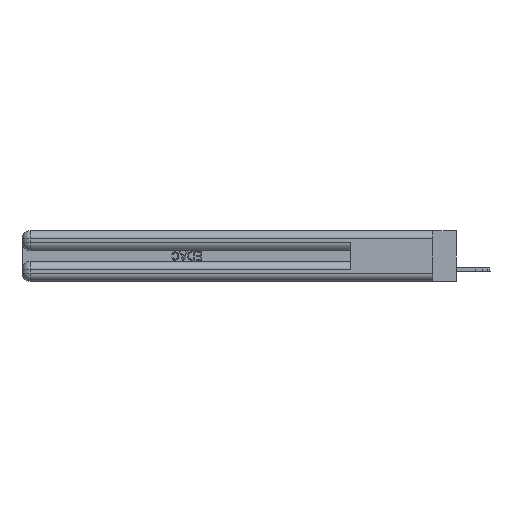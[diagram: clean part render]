
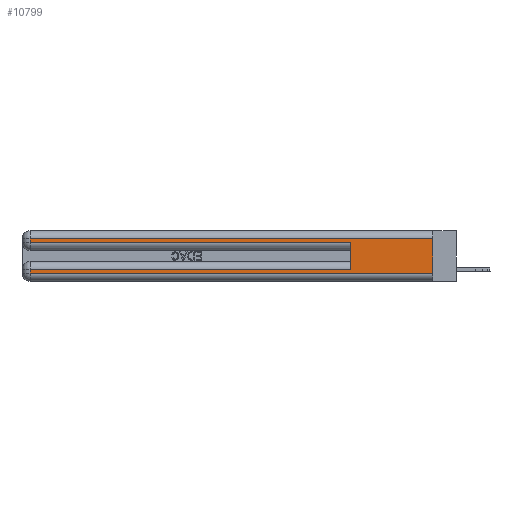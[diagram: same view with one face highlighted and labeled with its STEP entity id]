
A CAD part, left-side view. The second image highlights one B-rep face of the part: STEP entity #10799.
In plain terms, the highlighted planar face has unit normal (-1, 0, 0).
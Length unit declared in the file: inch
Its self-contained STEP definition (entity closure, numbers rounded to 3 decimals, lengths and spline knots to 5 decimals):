
#1402 = LINE ( 'NONE', #39074, #12026 ) ;
#1666 = ORIENTED_EDGE ( 'NONE', *, *, #37206, .F. ) ;
#1807 = PLANE ( 'NONE',  #17570 ) ;
#2458 = CARTESIAN_POINT ( 'NONE',  ( 0., 2.94, 0.06 ) ) ;
#2576 = CARTESIAN_POINT ( 'NONE',  ( 0., 0., 0.31 ) ) ;
#3632 = CARTESIAN_POINT ( 'NONE',  ( 0., 0., 0.085 ) ) ;
#4498 = LINE ( 'NONE', #38689, #5993 ) ;
#5146 = ORIENTED_EDGE ( 'NONE', *, *, #19513, .F. ) ;
#5199 = VERTEX_POINT ( 'NONE', #5343 ) ;
#5343 = CARTESIAN_POINT ( 'NONE',  ( 0., 2.94, 0.085 ) ) ;
#5422 = CARTESIAN_POINT ( 'NONE',  ( 0., 0., 0.37 ) ) ;
#5439 = ORIENTED_EDGE ( 'NONE', *, *, #12116, .T. ) ;
#5514 = CARTESIAN_POINT ( 'NONE',  ( 0., 0., 0.285 ) ) ;
#5993 = VECTOR ( 'NONE', #23153, 39.37008 ) ;
#6427 = VECTOR ( 'NONE', #16895, 39.37008 ) ;
#7506 = CARTESIAN_POINT ( 'NONE',  ( 0., 0., 0.31 ) ) ;
#7989 = DIRECTION ( 'NONE',  ( 0., 1., 0. ) ) ;
#9188 = VERTEX_POINT ( 'NONE', #35377 ) ;
#9248 = LINE ( 'NONE', #5422, #35304 ) ;
#9866 = VERTEX_POINT ( 'NONE', #32446 ) ;
#10028 = VECTOR ( 'NONE', #38394, 39.37008 ) ;
#10799 = ADVANCED_FACE ( 'NONE', ( #15548 ), #1807, .F. ) ;
#11138 = LINE ( 'NONE', #32343, #25615 ) ;
#12018 = VERTEX_POINT ( 'NONE', #26527 ) ;
#12026 = VECTOR ( 'NONE', #39212, 39.37008 ) ;
#12116 = EDGE_CURVE ( 'NONE', #9188, #5199, #19333, .T. ) ;
#13262 = VERTEX_POINT ( 'NONE', #38378 ) ;
#13413 = EDGE_CURVE ( 'NONE', #35289, #13262, #34206, .T. ) ;
#14549 = VERTEX_POINT ( 'NONE', #2458 ) ;
#14654 = DIRECTION ( 'NONE',  ( 0., 0., -1. ) ) ;
#15548 = FACE_OUTER_BOUND ( 'NONE', #35232, .T. ) ;
#16895 = DIRECTION ( 'NONE',  ( 0., -1., 0. ) ) ;
#17310 = EDGE_CURVE ( 'NONE', #14549, #12018, #4498, .T. ) ;
#17570 = AXIS2_PLACEMENT_3D ( 'NONE', #39318, #32699, #14654 ) ;
#18302 = CARTESIAN_POINT ( 'NONE',  ( 0., 0.6, 0.285 ) ) ;
#19301 = ORIENTED_EDGE ( 'NONE', *, *, #13413, .T. ) ;
#19333 = LINE ( 'NONE', #3632, #35766 ) ;
#19416 = ORIENTED_EDGE ( 'NONE', *, *, #37480, .T. ) ;
#19513 = EDGE_CURVE ( 'NONE', #9188, #36109, #1402, .T. ) ;
#21177 = ORIENTED_EDGE ( 'NONE', *, *, #17310, .T. ) ;
#21574 = VECTOR ( 'NONE', #34669, 39.37008 ) ;
#22087 = ORIENTED_EDGE ( 'NONE', *, *, #24289, .T. ) ;
#23153 = DIRECTION ( 'NONE',  ( 0., -1., 0. ) ) ;
#24142 = ORIENTED_EDGE ( 'NONE', *, *, #26947, .T. ) ;
#24289 = EDGE_CURVE ( 'NONE', #13262, #9866, #32673, .T. ) ;
#25615 = VECTOR ( 'NONE', #35332, 39.37008 ) ;
#26527 = CARTESIAN_POINT ( 'NONE',  ( 0., 0., 0.06 ) ) ;
#26947 = EDGE_CURVE ( 'NONE', #9866, #36109, #37300, .T. ) ;
#30360 = DIRECTION ( 'NONE',  ( 0., 0., -1. ) ) ;
#32343 = CARTESIAN_POINT ( 'NONE',  ( 0., 2.94, 0.37 ) ) ;
#32446 = CARTESIAN_POINT ( 'NONE',  ( 0., 2.94, 0.285 ) ) ;
#32673 = LINE ( 'NONE', #36987, #21574 ) ;
#32699 = DIRECTION ( 'NONE',  ( 1., 0., 0. ) ) ;
#34206 = LINE ( 'NONE', #7506, #10028 ) ;
#34669 = DIRECTION ( 'NONE',  ( 0., 0., -1. ) ) ;
#35232 = EDGE_LOOP ( 'NONE', ( #1666, #19301, #22087, #24142, #5146, #5439, #19416, #21177 ) ) ;
#35289 = VERTEX_POINT ( 'NONE', #2576 ) ;
#35304 = VECTOR ( 'NONE', #30360, 39.37008 ) ;
#35332 = DIRECTION ( 'NONE',  ( 0., 0., -1. ) ) ;
#35377 = CARTESIAN_POINT ( 'NONE',  ( 0., 0.6, 0.085 ) ) ;
#35766 = VECTOR ( 'NONE', #7989, 39.37008 ) ;
#36109 = VERTEX_POINT ( 'NONE', #18302 ) ;
#36987 = CARTESIAN_POINT ( 'NONE',  ( 0., 2.94, 0.37 ) ) ;
#37206 = EDGE_CURVE ( 'NONE', #35289, #12018, #9248, .T. ) ;
#37300 = LINE ( 'NONE', #5514, #6427 ) ;
#37480 = EDGE_CURVE ( 'NONE', #5199, #14549, #11138, .T. ) ;
#38378 = CARTESIAN_POINT ( 'NONE',  ( 0., 2.94, 0.31 ) ) ;
#38394 = DIRECTION ( 'NONE',  ( 0., 1., 0. ) ) ;
#38689 = CARTESIAN_POINT ( 'NONE',  ( 0., 0., 0.06 ) ) ;
#39074 = CARTESIAN_POINT ( 'NONE',  ( 0., 0.6, 0.145 ) ) ;
#39212 = DIRECTION ( 'NONE',  ( 0., 0., 1. ) ) ;
#39318 = CARTESIAN_POINT ( 'NONE',  ( 0., 0., 0.37 ) ) ;
